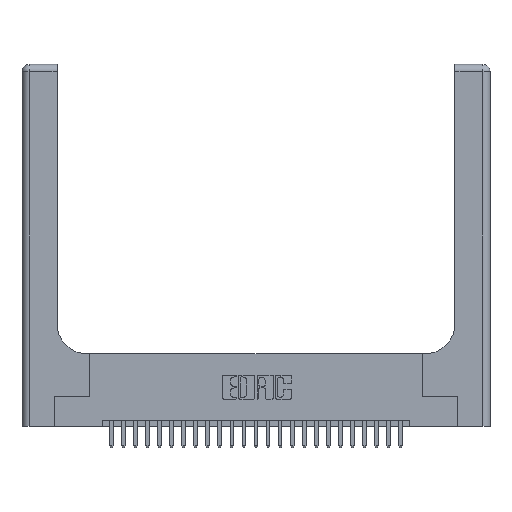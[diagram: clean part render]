
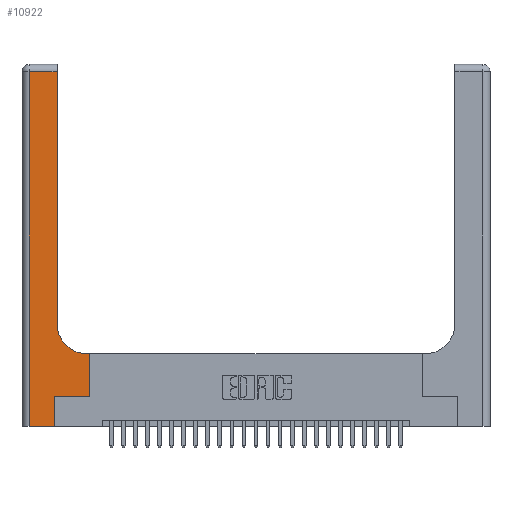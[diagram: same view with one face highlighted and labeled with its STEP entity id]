
A CAD part, top view. The second image highlights one B-rep face of the part: STEP entity #10922.
In plain terms, the highlighted planar face has unit normal (0, 0, 1).
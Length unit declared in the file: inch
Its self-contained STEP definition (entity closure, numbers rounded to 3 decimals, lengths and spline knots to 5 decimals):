
#40 = EDGE_LOOP ( 'NONE', ( #12621, #20305, #13583, #17802, #9050, #2542, #20081, #4553, #3647 ) ) ;
#299 = CARTESIAN_POINT ( 'NONE',  ( 0.269, 0.25, 0.37 ) ) ;
#418 = EDGE_CURVE ( 'NONE', #17581, #6298, #11773, .T. ) ;
#1227 = VECTOR ( 'NONE', #26935, 39.37008 ) ;
#1402 = VECTOR ( 'NONE', #7299, 39.37008 ) ;
#1675 = FACE_OUTER_BOUND ( 'NONE', #40, .T. ) ;
#1962 = VECTOR ( 'NONE', #23199, 39.37008 ) ;
#2245 = DIRECTION ( 'NONE',  ( 0., 1., 0. ) ) ;
#2373 = CARTESIAN_POINT ( 'NONE',  ( 0.06, 3., 0.37 ) ) ;
#2542 = ORIENTED_EDGE ( 'NONE', *, *, #5715, .T. ) ;
#3647 = ORIENTED_EDGE ( 'NONE', *, *, #4438, .T. ) ;
#3854 = CARTESIAN_POINT ( 'NONE',  ( 0.06, 0., 0.37 ) ) ;
#4127 = PLANE ( 'NONE',  #20539 ) ;
#4361 = CARTESIAN_POINT ( 'NONE',  ( 0., 2.94, 0.37 ) ) ;
#4438 = EDGE_CURVE ( 'NONE', #4685, #16559, #15981, .T. ) ;
#4553 = ORIENTED_EDGE ( 'NONE', *, *, #16610, .T. ) ;
#4554 = CARTESIAN_POINT ( 'NONE',  ( 0.2915, 3., 0.37 ) ) ;
#4685 = VERTEX_POINT ( 'NONE', #18098 ) ;
#5207 = LINE ( 'NONE', #4554, #21002 ) ;
#5397 = DIRECTION ( 'NONE',  ( 1., 0., 0. ) ) ;
#5715 = EDGE_CURVE ( 'NONE', #17613, #13646, #10403, .T. ) ;
#5746 = CARTESIAN_POINT ( 'NONE',  ( 0.269, 0.25, 0.37 ) ) ;
#6298 = VERTEX_POINT ( 'NONE', #15336 ) ;
#6419 = VECTOR ( 'NONE', #22506, 39.37008 ) ;
#7034 = DIRECTION ( 'NONE',  ( 0., -1., 0. ) ) ;
#7291 = EDGE_CURVE ( 'NONE', #6298, #15197, #24498, .T. ) ;
#7299 = DIRECTION ( 'NONE',  ( -1., 0., 0. ) ) ;
#9050 = ORIENTED_EDGE ( 'NONE', *, *, #15379, .T. ) ;
#9368 = VECTOR ( 'NONE', #7034, 39.37008 ) ;
#9652 = VERTEX_POINT ( 'NONE', #20553 ) ;
#10243 = CARTESIAN_POINT ( 'NONE',  ( 0., 0., 0.37 ) ) ;
#10335 = DIRECTION ( 'NONE',  ( -1., 0., 0. ) ) ;
#10403 = LINE ( 'NONE', #5746, #1227 ) ;
#10922 = ADVANCED_FACE ( 'NONE', ( #1675 ), #4127, .F. ) ;
#11578 = CARTESIAN_POINT ( 'NONE',  ( 0.5415, 0.85, 0.37 ) ) ;
#11743 = AXIS2_PLACEMENT_3D ( 'NONE', #11578, #17954, #5397 ) ;
#11773 = LINE ( 'NONE', #4361, #1962 ) ;
#12621 = ORIENTED_EDGE ( 'NONE', *, *, #25078, .T. ) ;
#12628 = LINE ( 'NONE', #16347, #6419 ) ;
#13085 = CARTESIAN_POINT ( 'NONE',  ( 0.2915, 0.85, 0.37 ) ) ;
#13583 = ORIENTED_EDGE ( 'NONE', *, *, #7291, .T. ) ;
#13646 = VERTEX_POINT ( 'NONE', #20301 ) ;
#14280 = VECTOR ( 'NONE', #17358, 39.37008 ) ;
#14826 = DIRECTION ( 'NONE',  ( 1., 0., 0. ) ) ;
#14972 = LINE ( 'NONE', #25888, #14280 ) ;
#15197 = VERTEX_POINT ( 'NONE', #3854 ) ;
#15336 = CARTESIAN_POINT ( 'NONE',  ( 0.06, 2.94, 0.37 ) ) ;
#15379 = EDGE_CURVE ( 'NONE', #25749, #17613, #14972, .T. ) ;
#15981 = CIRCLE ( 'NONE', #11743, 0.25 ) ;
#16347 = CARTESIAN_POINT ( 'NONE',  ( 0.5585, 0.25, 0.37 ) ) ;
#16420 = EDGE_CURVE ( 'NONE', #15197, #25749, #16842, .T. ) ;
#16559 = VERTEX_POINT ( 'NONE', #13085 ) ;
#16610 = EDGE_CURVE ( 'NONE', #9652, #4685, #26033, .T. ) ;
#16842 = LINE ( 'NONE', #10243, #19146 ) ;
#17358 = DIRECTION ( 'NONE',  ( 0., 1., 0. ) ) ;
#17581 = VERTEX_POINT ( 'NONE', #19117 ) ;
#17613 = VERTEX_POINT ( 'NONE', #299 ) ;
#17802 = ORIENTED_EDGE ( 'NONE', *, *, #16420, .T. ) ;
#17954 = DIRECTION ( 'NONE',  ( 0., 0., -1. ) ) ;
#18098 = CARTESIAN_POINT ( 'NONE',  ( 0.5415, 0.6, 0.37 ) ) ;
#19101 = DIRECTION ( 'NONE',  ( 0., 0., -1. ) ) ;
#19117 = CARTESIAN_POINT ( 'NONE',  ( 0.2915, 2.94, 0.37 ) ) ;
#19146 = VECTOR ( 'NONE', #14826, 39.37008 ) ;
#20081 = ORIENTED_EDGE ( 'NONE', *, *, #20252, .T. ) ;
#20252 = EDGE_CURVE ( 'NONE', #13646, #9652, #12628, .T. ) ;
#20301 = CARTESIAN_POINT ( 'NONE',  ( 0.5585, 0.25, 0.37 ) ) ;
#20305 = ORIENTED_EDGE ( 'NONE', *, *, #418, .T. ) ;
#20539 = AXIS2_PLACEMENT_3D ( 'NONE', #20965, #19101, #10335 ) ;
#20553 = CARTESIAN_POINT ( 'NONE',  ( 0.5585, 0.6, 0.37 ) ) ;
#20965 = CARTESIAN_POINT ( 'NONE',  ( 0., 3., 0.37 ) ) ;
#21002 = VECTOR ( 'NONE', #2245, 39.37008 ) ;
#22506 = DIRECTION ( 'NONE',  ( 0., 1., 0. ) ) ;
#23199 = DIRECTION ( 'NONE',  ( -1., 0., 0. ) ) ;
#23350 = CARTESIAN_POINT ( 'NONE',  ( 0.269, 0., 0.37 ) ) ;
#24498 = LINE ( 'NONE', #2373, #9368 ) ;
#25078 = EDGE_CURVE ( 'NONE', #16559, #17581, #5207, .T. ) ;
#25749 = VERTEX_POINT ( 'NONE', #23350 ) ;
#25888 = CARTESIAN_POINT ( 'NONE',  ( 0.269, 0., 0.37 ) ) ;
#26033 = LINE ( 'NONE', #26134, #1402 ) ;
#26134 = CARTESIAN_POINT ( 'NONE',  ( 0.2915, 0.6, 0.37 ) ) ;
#26935 = DIRECTION ( 'NONE',  ( 1., 0., 0. ) ) ;
